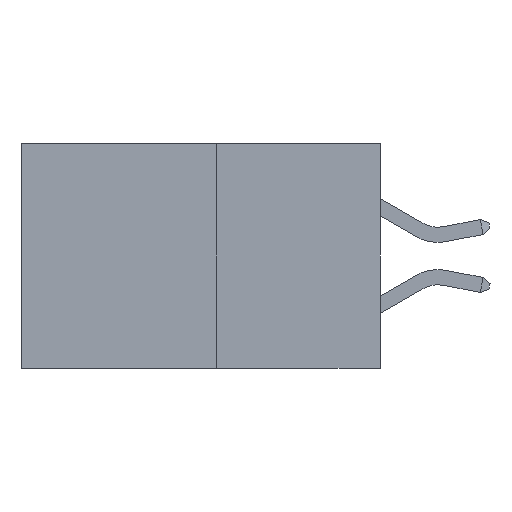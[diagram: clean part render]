
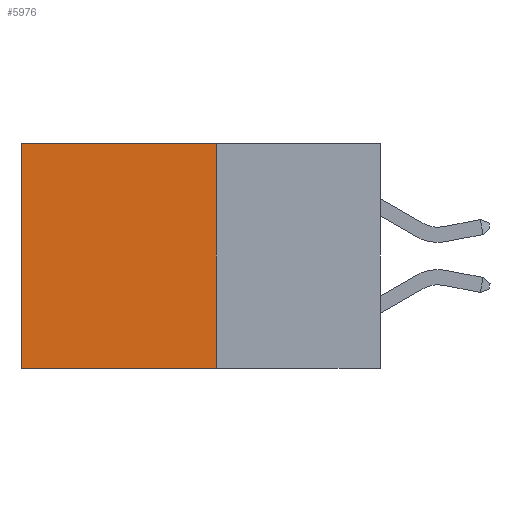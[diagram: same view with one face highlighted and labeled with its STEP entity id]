
A CAD part, left-side view. The second image highlights one B-rep face of the part: STEP entity #5976.
In plain terms, the highlighted planar face has unit normal (-1, 0, 0).
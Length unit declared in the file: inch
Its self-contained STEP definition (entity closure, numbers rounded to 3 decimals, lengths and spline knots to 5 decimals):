
#327 = LINE ( 'NONE', #6605, #3282 ) ;
#385 = AXIS2_PLACEMENT_3D ( 'NONE', #11309, #5613, #9523 ) ;
#613 = ORIENTED_EDGE ( 'NONE', *, *, #990, .T. ) ;
#912 = ORIENTED_EDGE ( 'NONE', *, *, #5413, .F. ) ;
#990 = EDGE_CURVE ( 'NONE', #11359, #10682, #9716, .T. ) ;
#1461 = VERTEX_POINT ( 'NONE', #7658 ) ;
#1790 = VECTOR ( 'NONE', #9874, 39.37008 ) ;
#3148 = CARTESIAN_POINT ( 'NONE',  ( 0.277, 0.27, -0.37 ) ) ;
#3282 = VECTOR ( 'NONE', #12402, 39.37008 ) ;
#3470 = FACE_OUTER_BOUND ( 'NONE', #5255, .T. ) ;
#3739 = DIRECTION ( 'NONE',  ( 0., 0., -1. ) ) ;
#3937 = VECTOR ( 'NONE', #3739, 39.37008 ) ;
#4177 = VERTEX_POINT ( 'NONE', #6992 ) ;
#4286 = PLANE ( 'NONE',  #385 ) ;
#4879 = DIRECTION ( 'NONE',  ( 0., 1., 0. ) ) ;
#5255 = EDGE_LOOP ( 'NONE', ( #613, #5933, #912, #11449 ) ) ;
#5413 = EDGE_CURVE ( 'NONE', #4177, #1461, #6652, .T. ) ;
#5419 = CARTESIAN_POINT ( 'NONE',  ( 0.277, 0.27, -0.37 ) ) ;
#5613 = DIRECTION ( 'NONE',  ( 1., 0., 0. ) ) ;
#5862 = CARTESIAN_POINT ( 'NONE',  ( 0.277, 0.59, 0. ) ) ;
#5933 = ORIENTED_EDGE ( 'NONE', *, *, #9245, .F. ) ;
#5976 = ADVANCED_FACE ( 'NONE', ( #3470 ), #4286, .F. ) ;
#6002 = CARTESIAN_POINT ( 'NONE',  ( 0.277, 0.59, -0.37 ) ) ;
#6605 = CARTESIAN_POINT ( 'NONE',  ( 0.277, 0.27, 0. ) ) ;
#6652 = LINE ( 'NONE', #5419, #3937 ) ;
#6992 = CARTESIAN_POINT ( 'NONE',  ( 0.277, 0.27, 0. ) ) ;
#7557 = LINE ( 'NONE', #3148, #9802 ) ;
#7658 = CARTESIAN_POINT ( 'NONE',  ( 0.277, 0.27, -0.37 ) ) ;
#9245 = EDGE_CURVE ( 'NONE', #1461, #10682, #7557, .T. ) ;
#9523 = DIRECTION ( 'NONE',  ( 0., 0., -1. ) ) ;
#9716 = LINE ( 'NONE', #6002, #1790 ) ;
#9802 = VECTOR ( 'NONE', #4879, 39.37008 ) ;
#9874 = DIRECTION ( 'NONE',  ( 0., 0., -1. ) ) ;
#10682 = VERTEX_POINT ( 'NONE', #11853 ) ;
#11111 = EDGE_CURVE ( 'NONE', #4177, #11359, #327, .T. ) ;
#11309 = CARTESIAN_POINT ( 'NONE',  ( 0.277, 0.27, -0.37 ) ) ;
#11359 = VERTEX_POINT ( 'NONE', #5862 ) ;
#11449 = ORIENTED_EDGE ( 'NONE', *, *, #11111, .T. ) ;
#11853 = CARTESIAN_POINT ( 'NONE',  ( 0.277, 0.59, -0.37 ) ) ;
#12402 = DIRECTION ( 'NONE',  ( 0., 1., 0. ) ) ;
